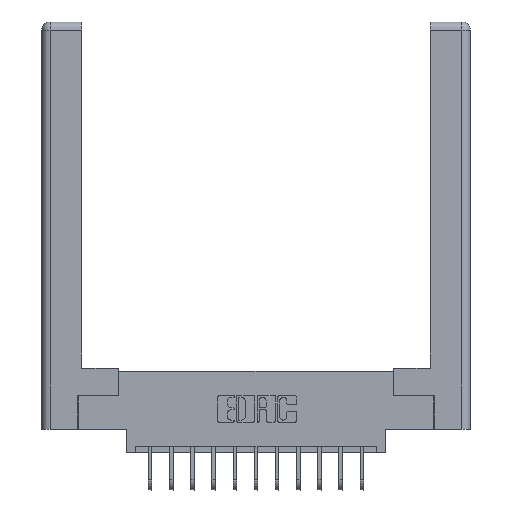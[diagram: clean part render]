
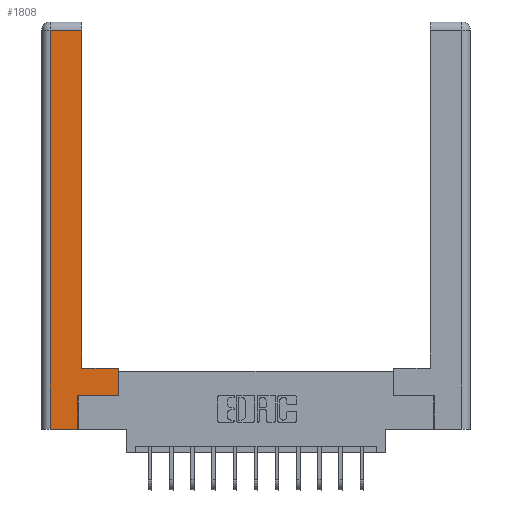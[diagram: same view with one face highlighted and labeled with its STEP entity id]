
A CAD part, top view. The second image highlights one B-rep face of the part: STEP entity #1808.
In plain terms, the highlighted planar face has unit normal (0, 0, 1).
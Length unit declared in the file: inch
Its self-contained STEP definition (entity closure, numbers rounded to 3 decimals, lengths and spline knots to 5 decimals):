
#371 = VECTOR ( 'NONE', #1258, 39.37008 ) ;
#468 = EDGE_CURVE ( 'NONE', #11220, #1001, #6457, .T. ) ;
#682 = VERTEX_POINT ( 'NONE', #14814 ) ;
#882 = ORIENTED_EDGE ( 'NONE', *, *, #13600, .T. ) ;
#1001 = VERTEX_POINT ( 'NONE', #9030 ) ;
#1156 = CARTESIAN_POINT ( 'NONE',  ( 0.295, 3., 0. ) ) ;
#1258 = DIRECTION ( 'NONE',  ( 0., 1., 0. ) ) ;
#1687 = CARTESIAN_POINT ( 'NONE',  ( 0.0615, 2.94, 0. ) ) ;
#1688 = EDGE_CURVE ( 'NONE', #13274, #11220, #5704, .T. ) ;
#1808 = ADVANCED_FACE ( 'NONE', ( #6418 ), #1989, .F. ) ;
#1989 = PLANE ( 'NONE',  #9148 ) ;
#2002 = LINE ( 'NONE', #3276, #6192 ) ;
#2235 = EDGE_CURVE ( 'NONE', #4291, #682, #13135, .T. ) ;
#2374 = ORIENTED_EDGE ( 'NONE', *, *, #3980, .T. ) ;
#2704 = CARTESIAN_POINT ( 'NONE',  ( 0.565, 0.245, 0. ) ) ;
#3084 = DIRECTION ( 'NONE',  ( 0., 1., 0. ) ) ;
#3179 = VECTOR ( 'NONE', #3084, 39.37008 ) ;
#3276 = CARTESIAN_POINT ( 'NONE',  ( 0.295, 0.45, 0. ) ) ;
#3816 = EDGE_CURVE ( 'NONE', #6685, #4291, #9821, .T. ) ;
#3866 = CARTESIAN_POINT ( 'NONE',  ( 0.565, 0.45, 0. ) ) ;
#3980 = EDGE_CURVE ( 'NONE', #14956, #7391, #2002, .T. ) ;
#4151 = ORIENTED_EDGE ( 'NONE', *, *, #7668, .T. ) ;
#4291 = VERTEX_POINT ( 'NONE', #8726 ) ;
#4599 = EDGE_CURVE ( 'NONE', #7391, #6685, #9791, .T. ) ;
#4994 = ORIENTED_EDGE ( 'NONE', *, *, #3816, .T. ) ;
#5448 = ORIENTED_EDGE ( 'NONE', *, *, #4599, .T. ) ;
#5470 = EDGE_LOOP ( 'NONE', ( #5448, #4994, #10244, #4151, #9119, #12309, #882, #2374 ) ) ;
#5541 = CARTESIAN_POINT ( 'NONE',  ( 0.565, 0.45, 0. ) ) ;
#5564 = DIRECTION ( 'NONE',  ( -1., 0., 0. ) ) ;
#5608 = DIRECTION ( 'NONE',  ( -1., 0., 0. ) ) ;
#5664 = VECTOR ( 'NONE', #5564, 39.37008 ) ;
#5704 = LINE ( 'NONE', #7564, #3179 ) ;
#6086 = CARTESIAN_POINT ( 'NONE',  ( 0.295, 2.94, 0. ) ) ;
#6192 = VECTOR ( 'NONE', #5608, 39.37008 ) ;
#6418 = FACE_OUTER_BOUND ( 'NONE', #5470, .T. ) ;
#6457 = LINE ( 'NONE', #2704, #12983 ) ;
#6685 = VERTEX_POINT ( 'NONE', #6086 ) ;
#6806 = DIRECTION ( 'NONE',  ( 0., 0., -1. ) ) ;
#7221 = CARTESIAN_POINT ( 'NONE',  ( 0.265, 0., 0. ) ) ;
#7391 = VERTEX_POINT ( 'NONE', #8679 ) ;
#7564 = CARTESIAN_POINT ( 'NONE',  ( 0.265, 0.245, 0. ) ) ;
#7668 = EDGE_CURVE ( 'NONE', #682, #13274, #11374, .T. ) ;
#8006 = CARTESIAN_POINT ( 'NONE',  ( 0.265, 0., 0. ) ) ;
#8625 = DIRECTION ( 'NONE',  ( 0., -1., 0. ) ) ;
#8679 = CARTESIAN_POINT ( 'NONE',  ( 0.295, 0.45, 0. ) ) ;
#8726 = CARTESIAN_POINT ( 'NONE',  ( 0.0615, 2.94, 0. ) ) ;
#8885 = VECTOR ( 'NONE', #13197, 39.37008 ) ;
#9030 = CARTESIAN_POINT ( 'NONE',  ( 0.565, 0.245, 0. ) ) ;
#9119 = ORIENTED_EDGE ( 'NONE', *, *, #1688, .T. ) ;
#9148 = AXIS2_PLACEMENT_3D ( 'NONE', #13670, #6806, #11327 ) ;
#9791 = LINE ( 'NONE', #1156, #371 ) ;
#9821 = LINE ( 'NONE', #1687, #5664 ) ;
#9931 = VECTOR ( 'NONE', #10678, 39.37008 ) ;
#10244 = ORIENTED_EDGE ( 'NONE', *, *, #2235, .T. ) ;
#10678 = DIRECTION ( 'NONE',  ( 1., 0., 0. ) ) ;
#11080 = LINE ( 'NONE', #3866, #8885 ) ;
#11143 = VECTOR ( 'NONE', #8625, 39.37008 ) ;
#11220 = VERTEX_POINT ( 'NONE', #12211 ) ;
#11327 = DIRECTION ( 'NONE',  ( -1., 0., 0. ) ) ;
#11374 = LINE ( 'NONE', #7221, #9931 ) ;
#12116 = CARTESIAN_POINT ( 'NONE',  ( 0.0615, 0., 0. ) ) ;
#12211 = CARTESIAN_POINT ( 'NONE',  ( 0.265, 0.245, 0. ) ) ;
#12309 = ORIENTED_EDGE ( 'NONE', *, *, #468, .T. ) ;
#12983 = VECTOR ( 'NONE', #13025, 39.37008 ) ;
#13025 = DIRECTION ( 'NONE',  ( 1., 0., 0. ) ) ;
#13135 = LINE ( 'NONE', #12116, #11143 ) ;
#13197 = DIRECTION ( 'NONE',  ( 0., 1., 0. ) ) ;
#13274 = VERTEX_POINT ( 'NONE', #8006 ) ;
#13600 = EDGE_CURVE ( 'NONE', #1001, #14956, #11080, .T. ) ;
#13670 = CARTESIAN_POINT ( 'NONE',  ( 0., 0., 0. ) ) ;
#14814 = CARTESIAN_POINT ( 'NONE',  ( 0.0615, 0., 0. ) ) ;
#14956 = VERTEX_POINT ( 'NONE', #5541 ) ;
